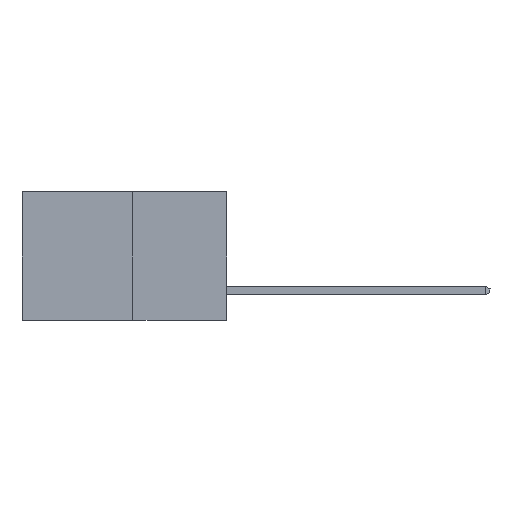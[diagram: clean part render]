
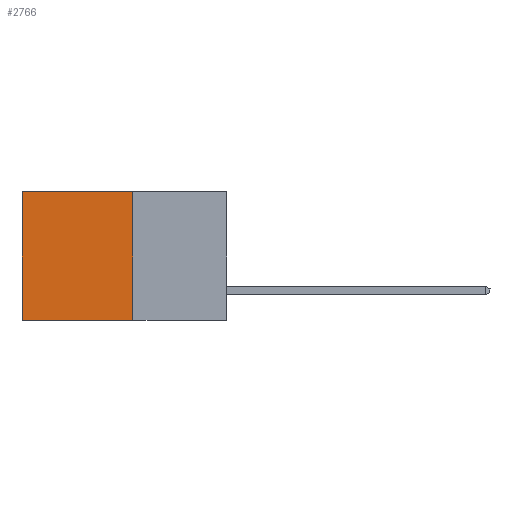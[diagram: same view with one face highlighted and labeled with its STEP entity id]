
A CAD part, left-side view. The second image highlights one B-rep face of the part: STEP entity #2766.
In plain terms, the highlighted planar face has unit normal (-1, 0, 0).
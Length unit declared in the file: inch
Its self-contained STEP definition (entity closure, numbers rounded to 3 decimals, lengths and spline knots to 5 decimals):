
#7 = CARTESIAN_POINT ( 'NONE',  ( 0.277, 0.27, 0. ) ) ;
#95 = CARTESIAN_POINT ( 'NONE',  ( 0.277, 0.27, -0.37 ) ) ;
#361 = CARTESIAN_POINT ( 'NONE',  ( 0.277, 0.27, -0.37 ) ) ;
#718 = CARTESIAN_POINT ( 'NONE',  ( 0.277, 0.27, 0. ) ) ;
#1286 = LINE ( 'NONE', #361, #1689 ) ;
#1689 = VECTOR ( 'NONE', #8301, 39.37008 ) ;
#2037 = DIRECTION ( 'NONE',  ( 0., 1., 0. ) ) ;
#2130 = DIRECTION ( 'NONE',  ( 0., 1., 0. ) ) ;
#2766 = ADVANCED_FACE ( 'NONE', ( #8194 ), #10945, .F. ) ;
#3047 = ORIENTED_EDGE ( 'NONE', *, *, #7550, .F. ) ;
#3147 = ORIENTED_EDGE ( 'NONE', *, *, #14972, .F. ) ;
#3157 = VERTEX_POINT ( 'NONE', #16572 ) ;
#3217 = ORIENTED_EDGE ( 'NONE', *, *, #14166, .T. ) ;
#3441 = VECTOR ( 'NONE', #3643, 39.37008 ) ;
#3643 = DIRECTION ( 'NONE',  ( 0., 0., -1. ) ) ;
#3725 = VERTEX_POINT ( 'NONE', #13136 ) ;
#4322 = ORIENTED_EDGE ( 'NONE', *, *, #5942, .T. ) ;
#4505 = VERTEX_POINT ( 'NONE', #15844 ) ;
#5942 = EDGE_CURVE ( 'NONE', #3725, #4505, #13319, .T. ) ;
#7550 = EDGE_CURVE ( 'NONE', #13854, #3157, #1286, .T. ) ;
#8194 = FACE_OUTER_BOUND ( 'NONE', #14169, .T. ) ;
#8301 = DIRECTION ( 'NONE',  ( 0., 0., -1. ) ) ;
#10583 = VECTOR ( 'NONE', #2130, 39.37008 ) ;
#10945 = PLANE ( 'NONE',  #11006 ) ;
#11006 = AXIS2_PLACEMENT_3D ( 'NONE', #95, #12645, #12441 ) ;
#11077 = LINE ( 'NONE', #718, #14001 ) ;
#12441 = DIRECTION ( 'NONE',  ( 0., 0., -1. ) ) ;
#12645 = DIRECTION ( 'NONE',  ( 1., 0., 0. ) ) ;
#13103 = LINE ( 'NONE', #13790, #10583 ) ;
#13136 = CARTESIAN_POINT ( 'NONE',  ( 0.277, 0.59, 0. ) ) ;
#13319 = LINE ( 'NONE', #15105, #3441 ) ;
#13790 = CARTESIAN_POINT ( 'NONE',  ( 0.277, 0.27, -0.37 ) ) ;
#13854 = VERTEX_POINT ( 'NONE', #7 ) ;
#14001 = VECTOR ( 'NONE', #2037, 39.37008 ) ;
#14166 = EDGE_CURVE ( 'NONE', #13854, #3725, #11077, .T. ) ;
#14169 = EDGE_LOOP ( 'NONE', ( #4322, #3147, #3047, #3217 ) ) ;
#14972 = EDGE_CURVE ( 'NONE', #3157, #4505, #13103, .T. ) ;
#15105 = CARTESIAN_POINT ( 'NONE',  ( 0.277, 0.59, -0.37 ) ) ;
#15844 = CARTESIAN_POINT ( 'NONE',  ( 0.277, 0.59, -0.37 ) ) ;
#16572 = CARTESIAN_POINT ( 'NONE',  ( 0.277, 0.27, -0.37 ) ) ;
